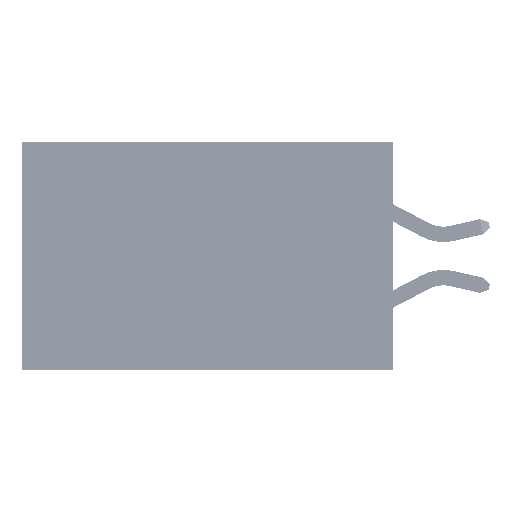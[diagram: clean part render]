
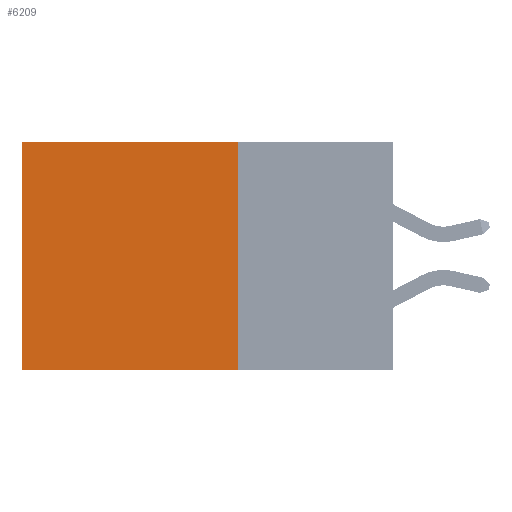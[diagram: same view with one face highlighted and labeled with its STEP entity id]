
A CAD part, left-side view. The second image highlights one B-rep face of the part: STEP entity #6209.
In plain terms, the highlighted planar face has unit normal (-1, 0, 0).
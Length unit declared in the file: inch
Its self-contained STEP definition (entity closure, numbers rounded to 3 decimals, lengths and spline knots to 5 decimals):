
#688 = DIRECTION ( 'NONE',  ( 0., 0., -1. ) ) ;
#4633 = FACE_OUTER_BOUND ( 'NONE', #26843, .T. ) ;
#6209 = ADVANCED_FACE ( 'NONE', ( #4633 ), #18827, .F. ) ;
#6283 = EDGE_CURVE ( 'NONE', #9768, #17692, #22556, .T. ) ;
#7909 = CARTESIAN_POINT ( 'NONE',  ( 0.2875, 0.25, 0. ) ) ;
#9768 = VERTEX_POINT ( 'NONE', #42189 ) ;
#10656 = ORIENTED_EDGE ( 'NONE', *, *, #6283, .T. ) ;
#11496 = CARTESIAN_POINT ( 'NONE',  ( 0.2875, 0.6, -0.37 ) ) ;
#11689 = VERTEX_POINT ( 'NONE', #27634 ) ;
#11809 = LINE ( 'NONE', #20670, #29958 ) ;
#13647 = VERTEX_POINT ( 'NONE', #11496 ) ;
#14824 = EDGE_CURVE ( 'NONE', #17692, #13647, #23335, .T. ) ;
#17692 = VERTEX_POINT ( 'NONE', #27527 ) ;
#18827 = PLANE ( 'NONE',  #39637 ) ;
#20047 = ORIENTED_EDGE ( 'NONE', *, *, #32665, .F. ) ;
#20670 = CARTESIAN_POINT ( 'NONE',  ( 0.2875, 0.25, -0.37 ) ) ;
#22556 = LINE ( 'NONE', #7909, #42582 ) ;
#23335 = LINE ( 'NONE', #41270, #42120 ) ;
#25955 = LINE ( 'NONE', #32948, #29481 ) ;
#26843 = EDGE_LOOP ( 'NONE', ( #33239, #32481, #20047, #10656 ) ) ;
#27527 = CARTESIAN_POINT ( 'NONE',  ( 0.2875, 0.6, 0. ) ) ;
#27634 = CARTESIAN_POINT ( 'NONE',  ( 0.2875, 0.25, -0.37 ) ) ;
#29331 = CARTESIAN_POINT ( 'NONE',  ( 0.2875, 0.25, 0. ) ) ;
#29481 = VECTOR ( 'NONE', #40407, 39.37008 ) ;
#29958 = VECTOR ( 'NONE', #38852, 39.37008 ) ;
#32481 = ORIENTED_EDGE ( 'NONE', *, *, #36205, .F. ) ;
#32665 = EDGE_CURVE ( 'NONE', #9768, #11689, #25955, .T. ) ;
#32948 = CARTESIAN_POINT ( 'NONE',  ( 0.2875, 0.25, 0. ) ) ;
#33045 = DIRECTION ( 'NONE',  ( 1., 0., 0. ) ) ;
#33239 = ORIENTED_EDGE ( 'NONE', *, *, #14824, .T. ) ;
#34060 = DIRECTION ( 'NONE',  ( 0., 0., -1. ) ) ;
#36205 = EDGE_CURVE ( 'NONE', #11689, #13647, #11809, .T. ) ;
#36775 = DIRECTION ( 'NONE',  ( 0., 1., 0. ) ) ;
#38852 = DIRECTION ( 'NONE',  ( 0., 1., 0. ) ) ;
#39637 = AXIS2_PLACEMENT_3D ( 'NONE', #29331, #33045, #688 ) ;
#40407 = DIRECTION ( 'NONE',  ( 0., 0., -1. ) ) ;
#41270 = CARTESIAN_POINT ( 'NONE',  ( 0.2875, 0.6, 0. ) ) ;
#42120 = VECTOR ( 'NONE', #34060, 39.37008 ) ;
#42189 = CARTESIAN_POINT ( 'NONE',  ( 0.2875, 0.25, 0. ) ) ;
#42582 = VECTOR ( 'NONE', #36775, 39.37008 ) ;
